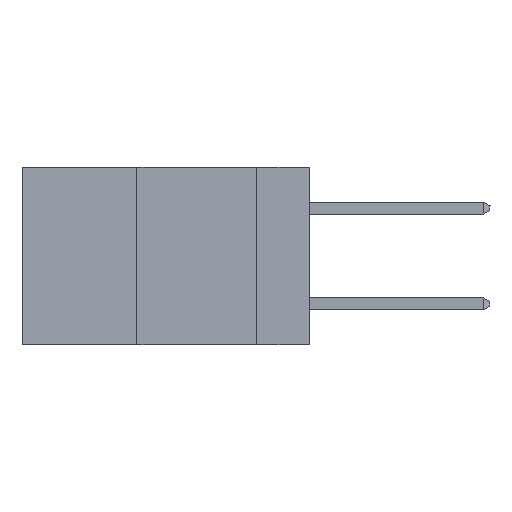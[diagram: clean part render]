
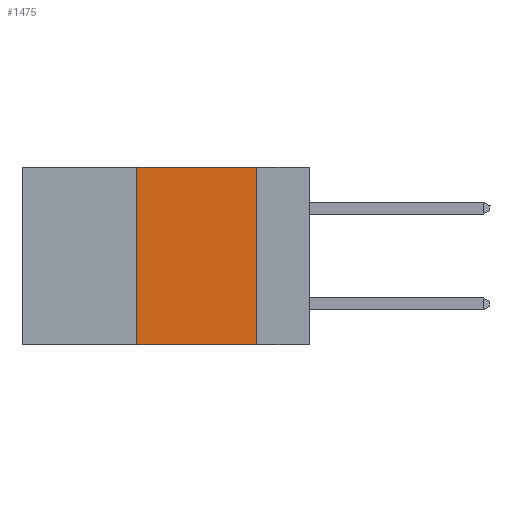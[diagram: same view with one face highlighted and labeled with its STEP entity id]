
A CAD part, left-side view. The second image highlights one B-rep face of the part: STEP entity #1475.
In plain terms, the highlighted planar face has unit normal (-1, 0, 0).
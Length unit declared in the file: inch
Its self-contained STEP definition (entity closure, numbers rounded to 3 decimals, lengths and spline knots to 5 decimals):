
#366 = LINE ( 'NONE', #24060, #2839 ) ;
#633 = VECTOR ( 'NONE', #25211, 39.37008 ) ;
#1475 = ADVANCED_FACE ( 'NONE', ( #28583 ), #4372, .F. ) ;
#2839 = VECTOR ( 'NONE', #16072, 39.37008 ) ;
#3605 = ORIENTED_EDGE ( 'NONE', *, *, #12643, .F. ) ;
#4172 = LINE ( 'NONE', #28026, #633 ) ;
#4372 = PLANE ( 'NONE',  #28167 ) ;
#5105 = EDGE_CURVE ( 'NONE', #5324, #24838, #25919, .T. ) ;
#5324 = VERTEX_POINT ( 'NONE', #24844 ) ;
#6580 = VERTEX_POINT ( 'NONE', #11793 ) ;
#8681 = CARTESIAN_POINT ( 'NONE',  ( 0., 0.6, 0. ) ) ;
#9481 = CARTESIAN_POINT ( 'NONE',  ( 0., 0.6, -0.37 ) ) ;
#10608 = LINE ( 'NONE', #31970, #32309 ) ;
#11169 = ORIENTED_EDGE ( 'NONE', *, *, #18172, .F. ) ;
#11793 = CARTESIAN_POINT ( 'NONE',  ( 0., 0.36, 0. ) ) ;
#12643 = EDGE_CURVE ( 'NONE', #5324, #6580, #4172, .T. ) ;
#14300 = VERTEX_POINT ( 'NONE', #29945 ) ;
#14370 = VECTOR ( 'NONE', #17761, 39.37008 ) ;
#16072 = DIRECTION ( 'NONE',  ( 0., 0., -1. ) ) ;
#17761 = DIRECTION ( 'NONE',  ( 0., -1., 0. ) ) ;
#18172 = EDGE_CURVE ( 'NONE', #14300, #24838, #366, .T. ) ;
#22225 = EDGE_CURVE ( 'NONE', #6580, #14300, #10608, .T. ) ;
#22753 = DIRECTION ( 'NONE',  ( 0., 0., -1. ) ) ;
#24060 = CARTESIAN_POINT ( 'NONE',  ( 0., 0.11, 0. ) ) ;
#24838 = VERTEX_POINT ( 'NONE', #25813 ) ;
#24844 = CARTESIAN_POINT ( 'NONE',  ( 0., 0.36, -0.37 ) ) ;
#25211 = DIRECTION ( 'NONE',  ( 0., 0., 1. ) ) ;
#25813 = CARTESIAN_POINT ( 'NONE',  ( 0., 0.11, -0.37 ) ) ;
#25919 = LINE ( 'NONE', #9481, #14370 ) ;
#26645 = ORIENTED_EDGE ( 'NONE', *, *, #5105, .T. ) ;
#27379 = ORIENTED_EDGE ( 'NONE', *, *, #22225, .F. ) ;
#28026 = CARTESIAN_POINT ( 'NONE',  ( 0., 0.36, 0. ) ) ;
#28167 = AXIS2_PLACEMENT_3D ( 'NONE', #8681, #31208, #22753 ) ;
#28583 = FACE_OUTER_BOUND ( 'NONE', #34231, .T. ) ;
#29945 = CARTESIAN_POINT ( 'NONE',  ( 0., 0.11, 0. ) ) ;
#31208 = DIRECTION ( 'NONE',  ( 1., 0., 0. ) ) ;
#31970 = CARTESIAN_POINT ( 'NONE',  ( 0., 0.6, 0. ) ) ;
#32309 = VECTOR ( 'NONE', #34612, 39.37008 ) ;
#34231 = EDGE_LOOP ( 'NONE', ( #11169, #27379, #3605, #26645 ) ) ;
#34612 = DIRECTION ( 'NONE',  ( 0., -1., 0. ) ) ;
